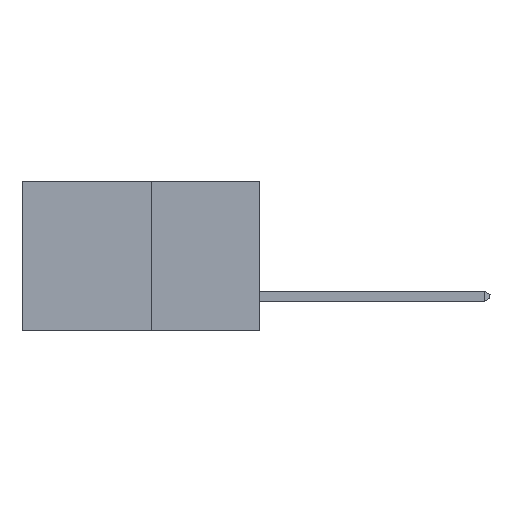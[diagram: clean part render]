
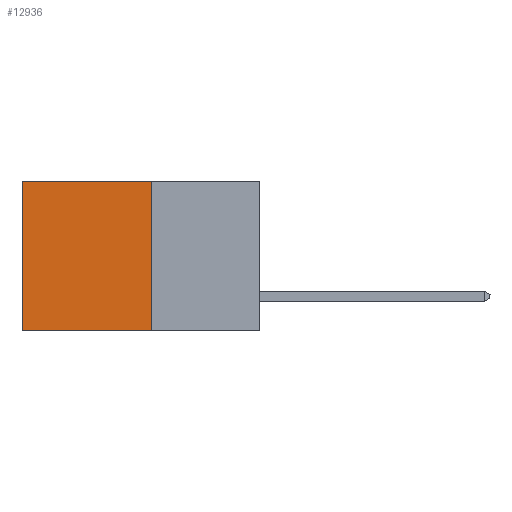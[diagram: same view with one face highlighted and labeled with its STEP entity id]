
A CAD part, left-side view. The second image highlights one B-rep face of the part: STEP entity #12936.
In plain terms, the highlighted planar face has unit normal (-1, 0, 0).
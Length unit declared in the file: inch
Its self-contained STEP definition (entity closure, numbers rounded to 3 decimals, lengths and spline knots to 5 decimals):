
#444 = CARTESIAN_POINT ( 'NONE',  ( 0.277, 0.27, -0.37 ) ) ;
#1071 = DIRECTION ( 'NONE',  ( 0., 1., 0. ) ) ;
#1474 = ORIENTED_EDGE ( 'NONE', *, *, #3520, .F. ) ;
#3520 = EDGE_CURVE ( 'NONE', #8636, #13654, #10244, .T. ) ;
#6347 = CARTESIAN_POINT ( 'NONE',  ( 0.277, 0.27, -0.37 ) ) ;
#8159 = DIRECTION ( 'NONE',  ( 0., 0., -1. ) ) ;
#8636 = VERTEX_POINT ( 'NONE', #10071 ) ;
#8692 = DIRECTION ( 'NONE',  ( 0., 0., -1. ) ) ;
#9695 = VECTOR ( 'NONE', #8692, 39.37008 ) ;
#9875 = VECTOR ( 'NONE', #11474, 39.37008 ) ;
#10071 = CARTESIAN_POINT ( 'NONE',  ( 0.277, 0.27, 0. ) ) ;
#10224 = CARTESIAN_POINT ( 'NONE',  ( 0.277, 0.27, 0. ) ) ;
#10244 = LINE ( 'NONE', #10353, #9695 ) ;
#10353 = CARTESIAN_POINT ( 'NONE',  ( 0.277, 0.27, -0.37 ) ) ;
#11474 = DIRECTION ( 'NONE',  ( 0., 0., -1. ) ) ;
#11521 = LINE ( 'NONE', #19823, #15559 ) ;
#11581 = ORIENTED_EDGE ( 'NONE', *, *, #21948, .F. ) ;
#12286 = LINE ( 'NONE', #10224, #16322 ) ;
#12704 = EDGE_LOOP ( 'NONE', ( #18464, #11581, #1474, #13175 ) ) ;
#12936 = ADVANCED_FACE ( 'NONE', ( #19905 ), #16851, .F. ) ;
#13175 = ORIENTED_EDGE ( 'NONE', *, *, #15814, .T. ) ;
#13654 = VERTEX_POINT ( 'NONE', #444 ) ;
#14881 = AXIS2_PLACEMENT_3D ( 'NONE', #6347, #18535, #8159 ) ;
#14946 = VERTEX_POINT ( 'NONE', #19899 ) ;
#15262 = CARTESIAN_POINT ( 'NONE',  ( 0.277, 0.59, -0.37 ) ) ;
#15559 = VECTOR ( 'NONE', #21510, 39.37008 ) ;
#15814 = EDGE_CURVE ( 'NONE', #8636, #14946, #12286, .T. ) ;
#16322 = VECTOR ( 'NONE', #1071, 39.37008 ) ;
#16779 = VERTEX_POINT ( 'NONE', #15262 ) ;
#16851 = PLANE ( 'NONE',  #14881 ) ;
#18271 = CARTESIAN_POINT ( 'NONE',  ( 0.277, 0.59, -0.37 ) ) ;
#18464 = ORIENTED_EDGE ( 'NONE', *, *, #22009, .T. ) ;
#18535 = DIRECTION ( 'NONE',  ( 1., 0., 0. ) ) ;
#19008 = LINE ( 'NONE', #18271, #9875 ) ;
#19823 = CARTESIAN_POINT ( 'NONE',  ( 0.277, 0.27, -0.37 ) ) ;
#19899 = CARTESIAN_POINT ( 'NONE',  ( 0.277, 0.59, 0. ) ) ;
#19905 = FACE_OUTER_BOUND ( 'NONE', #12704, .T. ) ;
#21510 = DIRECTION ( 'NONE',  ( 0., 1., 0. ) ) ;
#21948 = EDGE_CURVE ( 'NONE', #13654, #16779, #11521, .T. ) ;
#22009 = EDGE_CURVE ( 'NONE', #14946, #16779, #19008, .T. ) ;
